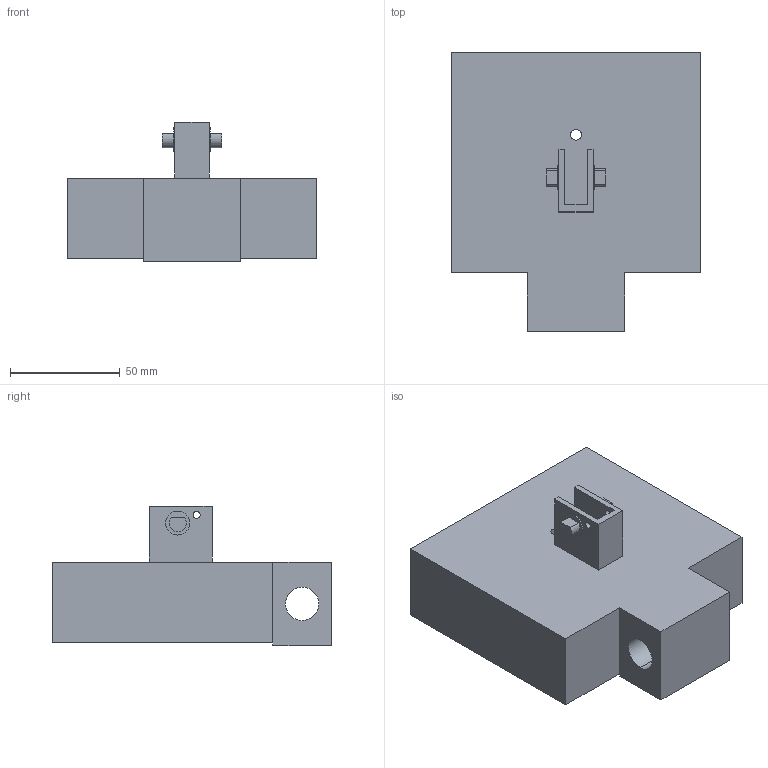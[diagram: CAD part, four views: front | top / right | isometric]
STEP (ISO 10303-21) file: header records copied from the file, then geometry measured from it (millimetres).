
FILE_DESCRIPTION (( 'STEP AP214' ), '1' );
FILE_NAME ('back_cover.STEP', '2013-09-07T19:08:56', ( '' ), ( '' ), 'SwSTEP 2.0', 'SolidWorks 2013', '' );
FILE_SCHEMA (( 'AUTOMOTIVE_DESIGN' ));
Length unit declared in the file: inch
Products named in the file (1): back_cover
Bounding box: 113.54 x 127 x 63.5 mm (x, y, z)
Volume: 460723.9 mm3; surface area: 49159.7 mm2
Topology: 1 solids, 1 shells, 42 faces, 103 edges, 68 vertices
Faces by surface type: plane 27, cylinder 15
Entity records: 1297 total; most frequent: DIRECTION 219, CARTESIAN_POINT 214, ORIENTED_EDGE 206, EDGE_CURVE 103, AXIS2_PLACEMENT_3D 73, VECTOR 73, LINE 73, VERTEX_POINT 68
